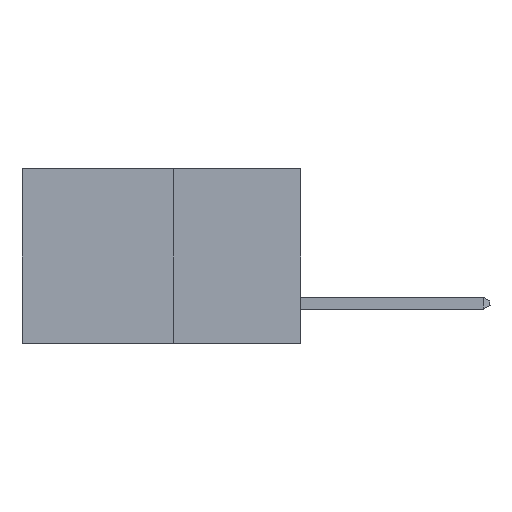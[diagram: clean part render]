
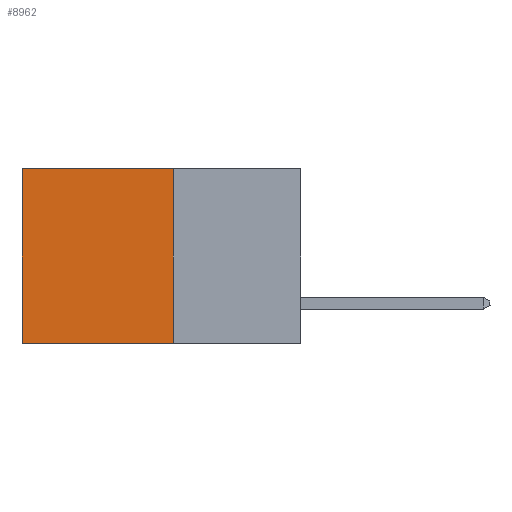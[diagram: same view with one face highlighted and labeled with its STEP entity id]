
A CAD part, left-side view. The second image highlights one B-rep face of the part: STEP entity #8962.
In plain terms, the highlighted planar face has unit normal (-1, 0, 0).
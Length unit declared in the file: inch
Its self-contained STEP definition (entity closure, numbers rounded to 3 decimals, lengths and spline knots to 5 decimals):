
#457 = CARTESIAN_POINT ( 'NONE',  ( 0.277, 0.27, 0. ) ) ;
#534 = CARTESIAN_POINT ( 'NONE',  ( 0.277, 0.59, -0.37 ) ) ;
#537 = CARTESIAN_POINT ( 'NONE',  ( 0.277, 0.27, -0.37 ) ) ;
#1760 = LINE ( 'NONE', #20846, #7996 ) ;
#1763 = VERTEX_POINT ( 'NONE', #8165 ) ;
#4332 = DIRECTION ( 'NONE',  ( 0., 0., -1. ) ) ;
#5587 = VECTOR ( 'NONE', #9763, 39.37008 ) ;
#6439 = CARTESIAN_POINT ( 'NONE',  ( 0.277, 0.59, 0. ) ) ;
#7202 = VECTOR ( 'NONE', #16509, 39.37008 ) ;
#7243 = DIRECTION ( 'NONE',  ( 0., 1., 0. ) ) ;
#7357 = EDGE_LOOP ( 'NONE', ( #28597, #26007, #28293, #13853 ) ) ;
#7939 = LINE ( 'NONE', #457, #7202 ) ;
#7996 = VECTOR ( 'NONE', #7243, 39.37008 ) ;
#8165 = CARTESIAN_POINT ( 'NONE',  ( 0.277, 0.27, 0. ) ) ;
#8962 = ADVANCED_FACE ( 'NONE', ( #24328 ), #15766, .F. ) ;
#9200 = DIRECTION ( 'NONE',  ( 0., 0., -1. ) ) ;
#9763 = DIRECTION ( 'NONE',  ( 0., 0., -1. ) ) ;
#10392 = EDGE_CURVE ( 'NONE', #1763, #17027, #7939, .T. ) ;
#12269 = EDGE_CURVE ( 'NONE', #17027, #22719, #23320, .T. ) ;
#13503 = CARTESIAN_POINT ( 'NONE',  ( 0.277, 0.27, -0.37 ) ) ;
#13853 = ORIENTED_EDGE ( 'NONE', *, *, #10392, .T. ) ;
#15766 = PLANE ( 'NONE',  #16570 ) ;
#16308 = CARTESIAN_POINT ( 'NONE',  ( 0.277, 0.27, -0.37 ) ) ;
#16509 = DIRECTION ( 'NONE',  ( 0., 1., 0. ) ) ;
#16570 = AXIS2_PLACEMENT_3D ( 'NONE', #13503, #18065, #4332 ) ;
#17027 = VERTEX_POINT ( 'NONE', #6439 ) ;
#18065 = DIRECTION ( 'NONE',  ( 1., 0., 0. ) ) ;
#19135 = EDGE_CURVE ( 'NONE', #26911, #22719, #1760, .T. ) ;
#20846 = CARTESIAN_POINT ( 'NONE',  ( 0.277, 0.27, -0.37 ) ) ;
#22604 = VECTOR ( 'NONE', #9200, 39.37008 ) ;
#22719 = VERTEX_POINT ( 'NONE', #534 ) ;
#23320 = LINE ( 'NONE', #29516, #22604 ) ;
#23736 = LINE ( 'NONE', #537, #5587 ) ;
#24328 = FACE_OUTER_BOUND ( 'NONE', #7357, .T. ) ;
#26007 = ORIENTED_EDGE ( 'NONE', *, *, #19135, .F. ) ;
#26911 = VERTEX_POINT ( 'NONE', #16308 ) ;
#28293 = ORIENTED_EDGE ( 'NONE', *, *, #29056, .F. ) ;
#28597 = ORIENTED_EDGE ( 'NONE', *, *, #12269, .T. ) ;
#29056 = EDGE_CURVE ( 'NONE', #1763, #26911, #23736, .T. ) ;
#29516 = CARTESIAN_POINT ( 'NONE',  ( 0.277, 0.59, -0.37 ) ) ;
